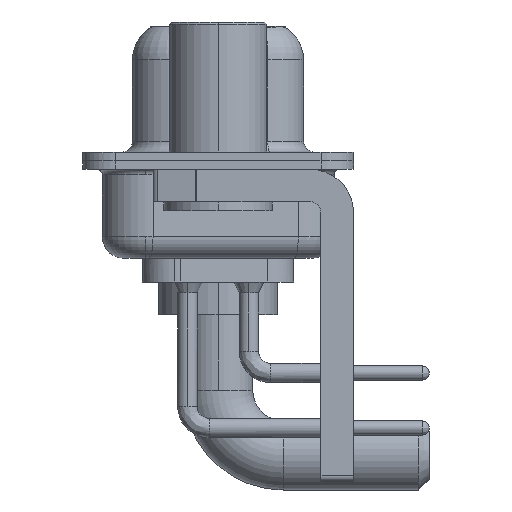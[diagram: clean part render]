
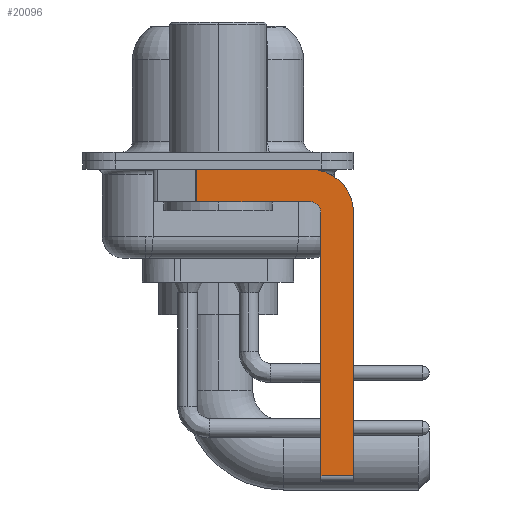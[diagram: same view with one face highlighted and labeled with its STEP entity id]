
A CAD part, left-side view. The second image highlights one B-rep face of the part: STEP entity #20096.
In plain terms, the highlighted planar face has unit normal (-1, 0, 0).
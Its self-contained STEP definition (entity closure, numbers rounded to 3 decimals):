
#62 = EDGE_CURVE ( 'NONE', #8509, #18183, #8659, .T. ) ;
#258 = LINE ( 'NONE', #14865, #5899 ) ;
#1159 = CARTESIAN_POINT ( 'NONE',  ( -2.9, 0.978, -0.4 ) ) ;
#1769 = AXIS2_PLACEMENT_3D ( 'NONE', #12289, #2438, #2536 ) ;
#2098 = ORIENTED_EDGE ( 'NONE', *, *, #2634, .T. ) ;
#2438 = DIRECTION ( 'NONE',  ( 1., 0., 0. ) ) ;
#2536 = DIRECTION ( 'NONE',  ( 0., 0., -1. ) ) ;
#2634 = EDGE_CURVE ( 'NONE', #19679, #16636, #8220, .T. ) ;
#2971 = ORIENTED_EDGE ( 'NONE', *, *, #19295, .F. ) ;
#3208 = VECTOR ( 'NONE', #17149, 1000. ) ;
#3431 = AXIS2_PLACEMENT_3D ( 'NONE', #5572, #4412, #12685 ) ;
#3790 = EDGE_CURVE ( 'NONE', #18712, #16636, #8598, .T. ) ;
#3936 = CARTESIAN_POINT ( 'NONE',  ( -2.9, -6.25, -14.55 ) ) ;
#4331 = CARTESIAN_POINT ( 'NONE',  ( -2.9, -6.25, -2.4 ) ) ;
#4412 = DIRECTION ( 'NONE',  ( 1., 0., 0. ) ) ;
#4419 = VECTOR ( 'NONE', #10483, 1000. ) ;
#4953 = CARTESIAN_POINT ( 'NONE',  ( -2.9, -4.25, -14.55 ) ) ;
#5453 = EDGE_CURVE ( 'NONE', #18681, #15063, #8128, .T. ) ;
#5572 = CARTESIAN_POINT ( 'NONE',  ( -2.9, -4.25, -2.4 ) ) ;
#5899 = VECTOR ( 'NONE', #11679, 1000. ) ;
#6072 = EDGE_CURVE ( 'NONE', #18681, #18183, #258, .T. ) ;
#6082 = ORIENTED_EDGE ( 'NONE', *, *, #5453, .F. ) ;
#6636 = DIRECTION ( 'NONE',  ( 0., -1., 0. ) ) ;
#6871 = ORIENTED_EDGE ( 'NONE', *, *, #6072, .T. ) ;
#6874 = VECTOR ( 'NONE', #11307, 1000. ) ;
#7009 = CARTESIAN_POINT ( 'NONE',  ( -2.9, -6.25, -2.4 ) ) ;
#7118 = ORIENTED_EDGE ( 'NONE', *, *, #18683, .F. ) ;
#7962 = EDGE_CURVE ( 'NONE', #17145, #8509, #9717, .T. ) ;
#8128 = LINE ( 'NONE', #20789, #6874 ) ;
#8220 = LINE ( 'NONE', #4953, #9730 ) ;
#8509 = VERTEX_POINT ( 'NONE', #10981 ) ;
#8598 = LINE ( 'NONE', #7009, #9828 ) ;
#8659 = LINE ( 'NONE', #19936, #3208 ) ;
#8888 = LINE ( 'NONE', #13986, #4419 ) ;
#9717 = CIRCLE ( 'NONE', #14846, 0.5 ) ;
#9730 = VECTOR ( 'NONE', #6636, 1000. ) ;
#9828 = VECTOR ( 'NONE', #15186, 1000. ) ;
#10483 = DIRECTION ( 'NONE',  ( 0., 0., 1. ) ) ;
#10702 = CARTESIAN_POINT ( 'NONE',  ( -2.9, -4.25, -2.4 ) ) ;
#10750 = CARTESIAN_POINT ( 'NONE',  ( -2.9, -4.75, -14.55 ) ) ;
#10823 = CARTESIAN_POINT ( 'NONE',  ( -2.9, 0.978, -1.9 ) ) ;
#10981 = CARTESIAN_POINT ( 'NONE',  ( -2.9, -4.25, -1.9 ) ) ;
#11307 = DIRECTION ( 'NONE',  ( 0., -1., 0. ) ) ;
#11679 = DIRECTION ( 'NONE',  ( 0., 0., -1. ) ) ;
#12289 = CARTESIAN_POINT ( 'NONE',  ( -2.9, -4.25, -2.4 ) ) ;
#12583 = CIRCLE ( 'NONE', #3431, 2. ) ;
#12685 = DIRECTION ( 'NONE',  ( 0., 0., -1. ) ) ;
#12776 = ORIENTED_EDGE ( 'NONE', *, *, #62, .F. ) ;
#13357 = CARTESIAN_POINT ( 'NONE',  ( -2.9, -4.75, -2.4 ) ) ;
#13479 = DIRECTION ( 'NONE',  ( -1., 0., 0. ) ) ;
#13986 = CARTESIAN_POINT ( 'NONE',  ( -2.9, -4.75, -14.8 ) ) ;
#14846 = AXIS2_PLACEMENT_3D ( 'NONE', #10702, #13479, #15170 ) ;
#14865 = CARTESIAN_POINT ( 'NONE',  ( -2.9, 0.978, -1.9 ) ) ;
#15063 = VERTEX_POINT ( 'NONE', #17717 ) ;
#15170 = DIRECTION ( 'NONE',  ( 0., 0., 1. ) ) ;
#15186 = DIRECTION ( 'NONE',  ( 0., 0., -1. ) ) ;
#15605 = EDGE_LOOP ( 'NONE', ( #6082, #6871, #12776, #20806, #7118, #2098, #16964, #2971 ) ) ;
#16636 = VERTEX_POINT ( 'NONE', #3936 ) ;
#16964 = ORIENTED_EDGE ( 'NONE', *, *, #3790, .F. ) ;
#16965 = FACE_OUTER_BOUND ( 'NONE', #15605, .T. ) ;
#17145 = VERTEX_POINT ( 'NONE', #13357 ) ;
#17149 = DIRECTION ( 'NONE',  ( 0., 1., 0. ) ) ;
#17279 = PLANE ( 'NONE',  #1769 ) ;
#17717 = CARTESIAN_POINT ( 'NONE',  ( -2.9, -4.25, -0.4 ) ) ;
#18183 = VERTEX_POINT ( 'NONE', #10823 ) ;
#18681 = VERTEX_POINT ( 'NONE', #1159 ) ;
#18683 = EDGE_CURVE ( 'NONE', #19679, #17145, #8888, .T. ) ;
#18712 = VERTEX_POINT ( 'NONE', #4331 ) ;
#19295 = EDGE_CURVE ( 'NONE', #15063, #18712, #12583, .T. ) ;
#19679 = VERTEX_POINT ( 'NONE', #10750 ) ;
#19936 = CARTESIAN_POINT ( 'NONE',  ( -2.9, -4.25, -1.9 ) ) ;
#20096 = ADVANCED_FACE ( 'NONE', ( #16965 ), #17279, .F. ) ;
#20789 = CARTESIAN_POINT ( 'NONE',  ( -2.9, 3., -0.4 ) ) ;
#20806 = ORIENTED_EDGE ( 'NONE', *, *, #7962, .F. ) ;
